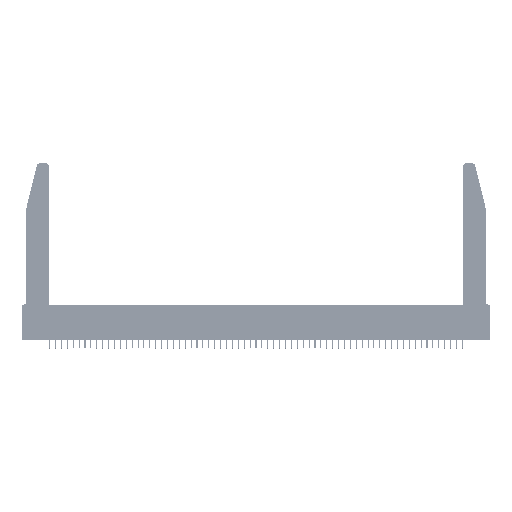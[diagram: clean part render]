
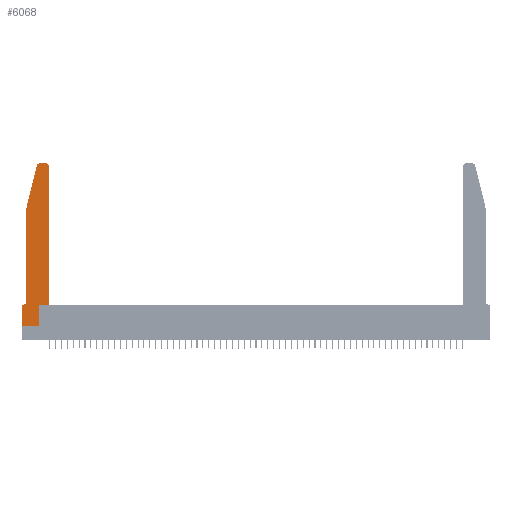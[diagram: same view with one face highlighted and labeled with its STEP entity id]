
A CAD part, top view. The second image highlights one B-rep face of the part: STEP entity #6068.
In plain terms, the highlighted planar face has unit normal (0, 0, 1).
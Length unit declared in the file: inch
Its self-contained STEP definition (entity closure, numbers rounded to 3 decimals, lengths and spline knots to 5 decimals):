
#911 = ORIENTED_EDGE ( 'NONE', *, *, #46708, .T. ) ;
#1281 = VERTEX_POINT ( 'NONE', #12561 ) ;
#2196 = DIRECTION ( 'NONE',  ( 1., 0., 0. ) ) ;
#2408 = DIRECTION ( 'NONE',  ( 0., 0., 1. ) ) ;
#2755 = VECTOR ( 'NONE', #33101, 39.37008 ) ;
#3189 = EDGE_CURVE ( 'NONE', #13786, #43617, #18815, .T. ) ;
#3414 = ORIENTED_EDGE ( 'NONE', *, *, #9586, .T. ) ;
#4239 = CARTESIAN_POINT ( 'NONE',  ( 0.4205, 2.72, 0.37 ) ) ;
#5225 = EDGE_CURVE ( 'NONE', #51982, #51334, #21636, .T. ) ;
#5327 = LINE ( 'NONE', #35728, #32191 ) ;
#5347 = CARTESIAN_POINT ( 'NONE',  ( 0.0755, 2., 0.37 ) ) ;
#6068 = ADVANCED_FACE ( 'NONE', ( #54701 ), #31768, .T. ) ;
#6376 = VERTEX_POINT ( 'NONE', #52098 ) ;
#8492 = ORIENTED_EDGE ( 'NONE', *, *, #5225, .T. ) ;
#9411 = VECTOR ( 'NONE', #21220, 39.37008 ) ;
#9494 = LINE ( 'NONE', #43640, #16251 ) ;
#9586 = EDGE_CURVE ( 'NONE', #43308, #31775, #36520, .T. ) ;
#9705 = ORIENTED_EDGE ( 'NONE', *, *, #33515, .T. ) ;
#11264 = CARTESIAN_POINT ( 'NONE',  ( 0.284, 2.72, 0.37 ) ) ;
#11557 = EDGE_CURVE ( 'NONE', #50032, #6376, #19895, .T. ) ;
#12561 = CARTESIAN_POINT ( 'NONE',  ( 0.4505, 0.35, 0.37 ) ) ;
#13101 = DIRECTION ( 'NONE',  ( 1., 0., 0. ) ) ;
#13341 = DIRECTION ( 'NONE',  ( 0., 1., 0. ) ) ;
#13786 = VERTEX_POINT ( 'NONE', #53552 ) ;
#14999 = ORIENTED_EDGE ( 'NONE', *, *, #11557, .T. ) ;
#15001 = CARTESIAN_POINT ( 'NONE',  ( 0., 0.35, 0.37 ) ) ;
#15084 = VECTOR ( 'NONE', #53544, 39.37008 ) ;
#16251 = VECTOR ( 'NONE', #26150, 39.37008 ) ;
#18668 = EDGE_CURVE ( 'NONE', #55440, #28676, #5327, .T. ) ;
#18815 = LINE ( 'NONE', #5347, #15084 ) ;
#19400 = DIRECTION ( 'NONE',  ( 0., 0., 1. ) ) ;
#19600 = DIRECTION ( 'NONE',  ( 1., 0., 0. ) ) ;
#19895 = LINE ( 'NONE', #37132, #2755 ) ;
#20898 = DIRECTION ( 'NONE',  ( -1., 0., 0. ) ) ;
#21091 = EDGE_CURVE ( 'NONE', #51334, #13786, #51827, .T. ) ;
#21220 = DIRECTION ( 'NONE',  ( 1., 0., 0. ) ) ;
#21636 = CIRCLE ( 'NONE', #38134, 0.03 ) ;
#22088 = LINE ( 'NONE', #43313, #9411 ) ;
#22246 = DIRECTION ( 'NONE',  ( -1., 0., 0. ) ) ;
#22833 = CARTESIAN_POINT ( 'NONE',  ( 0.4505, 0.35, 0.37 ) ) ;
#22925 = CARTESIAN_POINT ( 'NONE',  ( 0.2865, 0.35, 0.37 ) ) ;
#23337 = CARTESIAN_POINT ( 'NONE',  ( 0.0055, 0.35, 0.37 ) ) ;
#26150 = DIRECTION ( 'NONE',  ( 0., -1., 0. ) ) ;
#26431 = AXIS2_PLACEMENT_3D ( 'NONE', #4239, #31493, #13101 ) ;
#27103 = DIRECTION ( 'NONE',  ( -1., 0., 0. ) ) ;
#27627 = EDGE_CURVE ( 'NONE', #28676, #50032, #9494, .T. ) ;
#27971 = ORIENTED_EDGE ( 'NONE', *, *, #27627, .T. ) ;
#28676 = VERTEX_POINT ( 'NONE', #15001 ) ;
#30562 = VECTOR ( 'NONE', #56417, 39.37008 ) ;
#31392 = LINE ( 'NONE', #48898, #53526 ) ;
#31493 = DIRECTION ( 'NONE',  ( 0., 0., 1. ) ) ;
#31768 = PLANE ( 'NONE',  #56537 ) ;
#31775 = VERTEX_POINT ( 'NONE', #49792 ) ;
#32191 = VECTOR ( 'NONE', #22246, 39.37008 ) ;
#33101 = DIRECTION ( 'NONE',  ( 1., 0., 0. ) ) ;
#33515 = EDGE_CURVE ( 'NONE', #31775, #51982, #31392, .T. ) ;
#33540 = DIRECTION ( 'NONE',  ( 0., 0., -1. ) ) ;
#34897 = ORIENTED_EDGE ( 'NONE', *, *, #45487, .T. ) ;
#35046 = VERTEX_POINT ( 'NONE', #22925 ) ;
#35083 = ORIENTED_EDGE ( 'NONE', *, *, #18668, .T. ) ;
#35728 = CARTESIAN_POINT ( 'NONE',  ( 0.0755, 0.35, 0.37 ) ) ;
#36520 = CIRCLE ( 'NONE', #26431, 0.03 ) ;
#37132 = CARTESIAN_POINT ( 'NONE',  ( 0., 0., 0.37 ) ) ;
#37374 = ORIENTED_EDGE ( 'NONE', *, *, #3189, .T. ) ;
#38134 = AXIS2_PLACEMENT_3D ( 'NONE', #11264, #2408, #19600 ) ;
#38691 = CARTESIAN_POINT ( 'NONE',  ( 0.0055, 0.42, 0.37 ) ) ;
#38749 = ORIENTED_EDGE ( 'NONE', *, *, #51644, .T. ) ;
#40995 = ORIENTED_EDGE ( 'NONE', *, *, #21091, .T. ) ;
#41080 = ORIENTED_EDGE ( 'NONE', *, *, #49637, .T. ) ;
#42163 = LINE ( 'NONE', #43004, #51509 ) ;
#43004 = CARTESIAN_POINT ( 'NONE',  ( 0.2865, 0.35, 0.37 ) ) ;
#43250 = CARTESIAN_POINT ( 'NONE',  ( 0., 0., 0.37 ) ) ;
#43308 = VERTEX_POINT ( 'NONE', #52816 ) ;
#43313 = CARTESIAN_POINT ( 'NONE',  ( 0.4505, 0.35, 0.37 ) ) ;
#43617 = VERTEX_POINT ( 'NONE', #51593 ) ;
#43640 = CARTESIAN_POINT ( 'NONE',  ( 0., 0., 0.37 ) ) ;
#43925 = CARTESIAN_POINT ( 'NONE',  ( 0.25487, 2.72718, 0.37 ) ) ;
#44891 = AXIS2_PLACEMENT_3D ( 'NONE', #38691, #33540, #20898 ) ;
#45487 = EDGE_CURVE ( 'NONE', #1281, #43308, #52964, .T. ) ;
#45519 = CARTESIAN_POINT ( 'NONE',  ( 0., 0.35, 0.37 ) ) ;
#46708 = EDGE_CURVE ( 'NONE', #43617, #55440, #54085, .T. ) ;
#46759 = DIRECTION ( 'NONE',  ( 0., 1., 0. ) ) ;
#47541 = VECTOR ( 'NONE', #13341, 39.37008 ) ;
#47795 = CARTESIAN_POINT ( 'NONE',  ( 0.0755, 2., 0.37 ) ) ;
#48866 = EDGE_LOOP ( 'NONE', ( #9705, #8492, #40995, #37374, #911, #35083, #27971, #14999, #38749, #41080, #34897, #3414 ) ) ;
#48898 = CARTESIAN_POINT ( 'NONE',  ( 0.2605, 2.75, 0.37 ) ) ;
#49637 = EDGE_CURVE ( 'NONE', #35046, #1281, #22088, .T. ) ;
#49792 = CARTESIAN_POINT ( 'NONE',  ( 0.4205, 2.75, 0.37 ) ) ;
#50032 = VERTEX_POINT ( 'NONE', #43250 ) ;
#51334 = VERTEX_POINT ( 'NONE', #43925 ) ;
#51509 = VECTOR ( 'NONE', #46759, 39.37008 ) ;
#51593 = CARTESIAN_POINT ( 'NONE',  ( 0.0755, 0.42, 0.37 ) ) ;
#51644 = EDGE_CURVE ( 'NONE', #6376, #35046, #42163, .T. ) ;
#51827 = LINE ( 'NONE', #47795, #30562 ) ;
#51982 = VERTEX_POINT ( 'NONE', #53904 ) ;
#52098 = CARTESIAN_POINT ( 'NONE',  ( 0.2865, 0., 0.37 ) ) ;
#52816 = CARTESIAN_POINT ( 'NONE',  ( 0.4505, 2.72, 0.37 ) ) ;
#52964 = LINE ( 'NONE', #22833, #47541 ) ;
#53526 = VECTOR ( 'NONE', #27103, 39.37008 ) ;
#53544 = DIRECTION ( 'NONE',  ( 0., -1., 0. ) ) ;
#53552 = CARTESIAN_POINT ( 'NONE',  ( 0.0755, 2., 0.37 ) ) ;
#53904 = CARTESIAN_POINT ( 'NONE',  ( 0.284, 2.75, 0.37 ) ) ;
#54085 = CIRCLE ( 'NONE', #44891, 0.07 ) ;
#54701 = FACE_OUTER_BOUND ( 'NONE', #48866, .T. ) ;
#55440 = VERTEX_POINT ( 'NONE', #23337 ) ;
#56417 = DIRECTION ( 'NONE',  ( -0.239, -0.971, 0. ) ) ;
#56537 = AXIS2_PLACEMENT_3D ( 'NONE', #45519, #19400, #2196 ) ;
